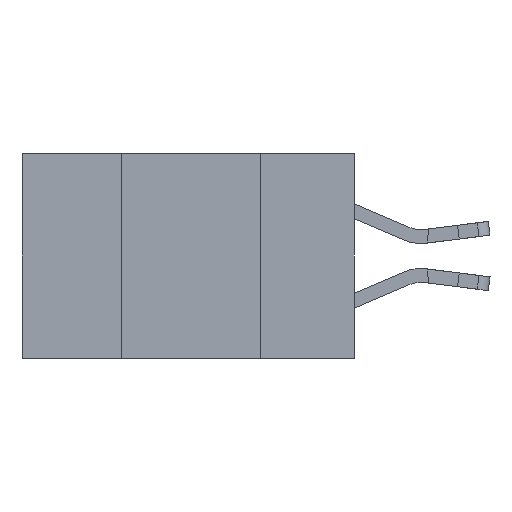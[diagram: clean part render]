
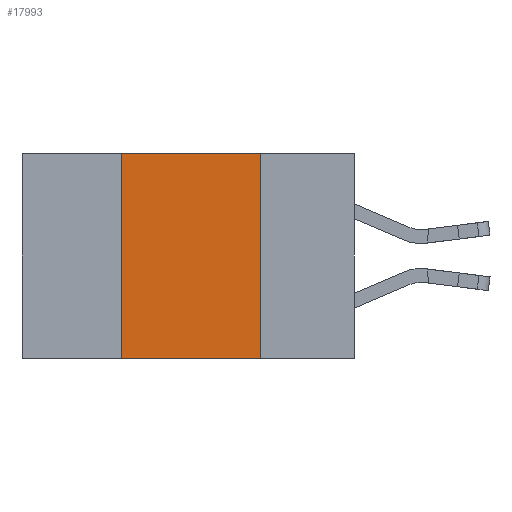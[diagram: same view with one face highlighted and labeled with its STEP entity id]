
A CAD part, left-side view. The second image highlights one B-rep face of the part: STEP entity #17993.
In plain terms, the highlighted planar face has unit normal (-1, 0, 0).
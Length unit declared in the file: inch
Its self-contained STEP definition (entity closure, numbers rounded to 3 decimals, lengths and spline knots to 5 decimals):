
#681 = EDGE_CURVE ( 'NONE', #5521, #9144, #6439, .T. ) ;
#1475 = DIRECTION ( 'NONE',  ( 0., 0., -1. ) ) ;
#1968 = EDGE_CURVE ( 'NONE', #6856, #5521, #4344, .T. ) ;
#3200 = CARTESIAN_POINT ( 'NONE',  ( 0., 0.42, 0. ) ) ;
#3696 = FACE_OUTER_BOUND ( 'NONE', #6975, .T. ) ;
#3921 = CARTESIAN_POINT ( 'NONE',  ( 0., 0.17, -0.37 ) ) ;
#4344 = LINE ( 'NONE', #16763, #17159 ) ;
#4619 = DIRECTION ( 'NONE',  ( 0., 0., 1. ) ) ;
#5521 = VERTEX_POINT ( 'NONE', #9742 ) ;
#5693 = EDGE_CURVE ( 'NONE', #14554, #6856, #15054, .T. ) ;
#5775 = LINE ( 'NONE', #17344, #18499 ) ;
#6439 = LINE ( 'NONE', #17218, #14991 ) ;
#6856 = VERTEX_POINT ( 'NONE', #3200 ) ;
#6975 = EDGE_LOOP ( 'NONE', ( #20666, #14338, #16306, #19075 ) ) ;
#8350 = DIRECTION ( 'NONE',  ( 0., -1., 0. ) ) ;
#9121 = VECTOR ( 'NONE', #4619, 39.37008 ) ;
#9144 = VERTEX_POINT ( 'NONE', #3921 ) ;
#9423 = EDGE_CURVE ( 'NONE', #14554, #9144, #5775, .T. ) ;
#9742 = CARTESIAN_POINT ( 'NONE',  ( 0., 0.17, 0. ) ) ;
#10702 = PLANE ( 'NONE',  #17508 ) ;
#11017 = CARTESIAN_POINT ( 'NONE',  ( 0., 0.42, -0.37 ) ) ;
#12510 = DIRECTION ( 'NONE',  ( 1., 0., 0. ) ) ;
#14338 = ORIENTED_EDGE ( 'NONE', *, *, #1968, .F. ) ;
#14554 = VERTEX_POINT ( 'NONE', #11017 ) ;
#14991 = VECTOR ( 'NONE', #17682, 39.37008 ) ;
#15054 = LINE ( 'NONE', #19049, #9121 ) ;
#16306 = ORIENTED_EDGE ( 'NONE', *, *, #5693, .F. ) ;
#16712 = DIRECTION ( 'NONE',  ( 0., -1., 0. ) ) ;
#16763 = CARTESIAN_POINT ( 'NONE',  ( 0., 0.6, 0. ) ) ;
#17159 = VECTOR ( 'NONE', #16712, 39.37008 ) ;
#17218 = CARTESIAN_POINT ( 'NONE',  ( 0., 0.17, -0.37 ) ) ;
#17344 = CARTESIAN_POINT ( 'NONE',  ( 0., 0.6, -0.37 ) ) ;
#17508 = AXIS2_PLACEMENT_3D ( 'NONE', #23171, #12510, #1475 ) ;
#17682 = DIRECTION ( 'NONE',  ( 0., 0., -1. ) ) ;
#17993 = ADVANCED_FACE ( 'NONE', ( #3696 ), #10702, .F. ) ;
#18499 = VECTOR ( 'NONE', #8350, 39.37008 ) ;
#19049 = CARTESIAN_POINT ( 'NONE',  ( 0., 0.42, -0.37 ) ) ;
#19075 = ORIENTED_EDGE ( 'NONE', *, *, #9423, .T. ) ;
#20666 = ORIENTED_EDGE ( 'NONE', *, *, #681, .F. ) ;
#23171 = CARTESIAN_POINT ( 'NONE',  ( 0., 0.6, 0. ) ) ;
